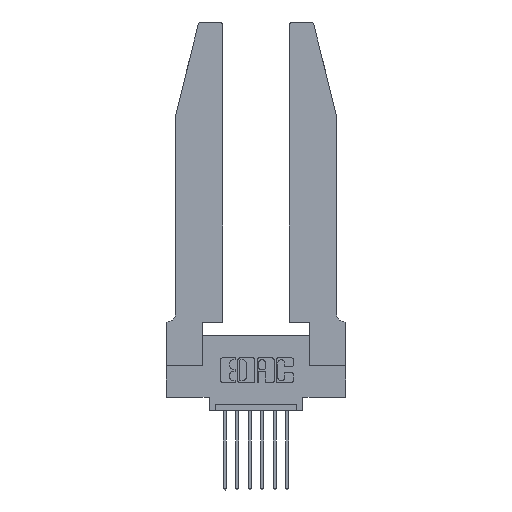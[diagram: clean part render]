
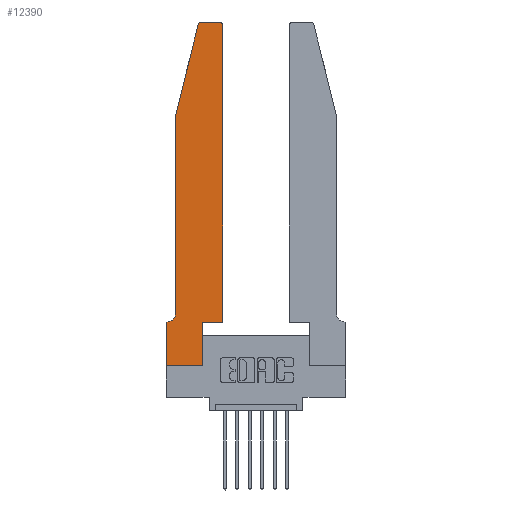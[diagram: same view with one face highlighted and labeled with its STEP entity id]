
A CAD part, top view. The second image highlights one B-rep face of the part: STEP entity #12390.
In plain terms, the highlighted planar face has unit normal (0, 0, 1).
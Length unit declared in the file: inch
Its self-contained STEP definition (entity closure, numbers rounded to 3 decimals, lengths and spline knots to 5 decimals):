
#160 = CARTESIAN_POINT ( 'NONE',  ( 0., 0.35, 0.37 ) ) ;
#162 = DIRECTION ( 'NONE',  ( -1., 0., 0. ) ) ;
#204 = PLANE ( 'NONE',  #5312 ) ;
#361 = DIRECTION ( 'NONE',  ( 1., 0., 0. ) ) ;
#409 = DIRECTION ( 'NONE',  ( 0., 0., 1. ) ) ;
#435 = VERTEX_POINT ( 'NONE', #12884 ) ;
#530 = CIRCLE ( 'NONE', #12871, 0.03 ) ;
#577 = DIRECTION ( 'NONE',  ( 1., 0., 0. ) ) ;
#799 = VERTEX_POINT ( 'NONE', #11457 ) ;
#1276 = LINE ( 'NONE', #7693, #9684 ) ;
#1311 = DIRECTION ( 'NONE',  ( -1., 0., 0. ) ) ;
#1637 = CARTESIAN_POINT ( 'NONE',  ( 0.284, 2.72, 0.37 ) ) ;
#1907 = ORIENTED_EDGE ( 'NONE', *, *, #7547, .T. ) ;
#2200 = VERTEX_POINT ( 'NONE', #2783 ) ;
#2266 = ORIENTED_EDGE ( 'NONE', *, *, #13866, .T. ) ;
#2279 = CIRCLE ( 'NONE', #2395, 0.07 ) ;
#2322 = VECTOR ( 'NONE', #10200, 39.37008 ) ;
#2341 = LINE ( 'NONE', #8963, #13403 ) ;
#2395 = AXIS2_PLACEMENT_3D ( 'NONE', #3370, #12209, #4284 ) ;
#2571 = EDGE_CURVE ( 'NONE', #3270, #6875, #530, .T. ) ;
#2683 = LINE ( 'NONE', #4864, #9753 ) ;
#2771 = DIRECTION ( 'NONE',  ( 1., 0., 0. ) ) ;
#2783 = CARTESIAN_POINT ( 'NONE',  ( 0.0055, 0.35, 0.37 ) ) ;
#3173 = VERTEX_POINT ( 'NONE', #13539 ) ;
#3248 = CARTESIAN_POINT ( 'NONE',  ( 0.4205, 2.75, 0.37 ) ) ;
#3270 = VERTEX_POINT ( 'NONE', #7578 ) ;
#3309 = CARTESIAN_POINT ( 'NONE',  ( 0., 0., 0.37 ) ) ;
#3370 = CARTESIAN_POINT ( 'NONE',  ( 0.0055, 0.42, 0.37 ) ) ;
#3454 = CARTESIAN_POINT ( 'NONE',  ( 0.0755, 0.42, 0.37 ) ) ;
#3624 = VECTOR ( 'NONE', #6893, 39.37008 ) ;
#3678 = CARTESIAN_POINT ( 'NONE',  ( 0., 0., 0.37 ) ) ;
#4079 = CARTESIAN_POINT ( 'NONE',  ( 0.0755, 2., 0.37 ) ) ;
#4284 = DIRECTION ( 'NONE',  ( -1., 0., 0. ) ) ;
#4397 = VECTOR ( 'NONE', #1311, 39.37008 ) ;
#4595 = DIRECTION ( 'NONE',  ( 1., 0., 0. ) ) ;
#4669 = EDGE_CURVE ( 'NONE', #2200, #3173, #7354, .T. ) ;
#4854 = VERTEX_POINT ( 'NONE', #3678 ) ;
#4864 = CARTESIAN_POINT ( 'NONE',  ( 0.4505, 0.35, 0.37 ) ) ;
#4888 = CARTESIAN_POINT ( 'NONE',  ( 0.4205, 2.72, 0.37 ) ) ;
#4927 = EDGE_CURVE ( 'NONE', #435, #7737, #2683, .T. ) ;
#5223 = VECTOR ( 'NONE', #4595, 39.37008 ) ;
#5266 = ORIENTED_EDGE ( 'NONE', *, *, #9468, .T. ) ;
#5312 = AXIS2_PLACEMENT_3D ( 'NONE', #160, #10130, #11325 ) ;
#5315 = LINE ( 'NONE', #10789, #8556 ) ;
#5510 = EDGE_CURVE ( 'NONE', #3173, #4854, #10440, .T. ) ;
#5637 = ORIENTED_EDGE ( 'NONE', *, *, #2571, .T. ) ;
#5814 = ORIENTED_EDGE ( 'NONE', *, *, #4927, .T. ) ;
#6471 = VERTEX_POINT ( 'NONE', #3248 ) ;
#6473 = ORIENTED_EDGE ( 'NONE', *, *, #7087, .T. ) ;
#6847 = CARTESIAN_POINT ( 'NONE',  ( 0.4505, 0.35, 0.37 ) ) ;
#6875 = VERTEX_POINT ( 'NONE', #13469 ) ;
#6893 = DIRECTION ( 'NONE',  ( 0., 1., 0. ) ) ;
#7062 = FACE_OUTER_BOUND ( 'NONE', #13129, .T. ) ;
#7087 = EDGE_CURVE ( 'NONE', #9486, #2200, #2279, .T. ) ;
#7101 = CIRCLE ( 'NONE', #13551, 0.03 ) ;
#7314 = ORIENTED_EDGE ( 'NONE', *, *, #9556, .T. ) ;
#7354 = LINE ( 'NONE', #7534, #4397 ) ;
#7426 = LINE ( 'NONE', #6847, #3624 ) ;
#7534 = CARTESIAN_POINT ( 'NONE',  ( 0.0755, 0.35, 0.37 ) ) ;
#7547 = EDGE_CURVE ( 'NONE', #7737, #10985, #7426, .T. ) ;
#7578 = CARTESIAN_POINT ( 'NONE',  ( 0.284, 2.75, 0.37 ) ) ;
#7693 = CARTESIAN_POINT ( 'NONE',  ( 0.2605, 2.75, 0.37 ) ) ;
#7723 = EDGE_CURVE ( 'NONE', #8467, #9486, #11390, .T. ) ;
#7737 = VERTEX_POINT ( 'NONE', #10017 ) ;
#7788 = LINE ( 'NONE', #3309, #5223 ) ;
#7909 = DIRECTION ( 'NONE',  ( -0.239, -0.971, 0. ) ) ;
#8229 = DIRECTION ( 'NONE',  ( 0., 0., 1. ) ) ;
#8467 = VERTEX_POINT ( 'NONE', #10449 ) ;
#8556 = VECTOR ( 'NONE', #13033, 39.37008 ) ;
#8605 = ORIENTED_EDGE ( 'NONE', *, *, #4669, .T. ) ;
#8676 = ORIENTED_EDGE ( 'NONE', *, *, #12314, .T. ) ;
#8781 = ORIENTED_EDGE ( 'NONE', *, *, #5510, .T. ) ;
#8963 = CARTESIAN_POINT ( 'NONE',  ( 0.0755, 2., 0.37 ) ) ;
#9336 = ORIENTED_EDGE ( 'NONE', *, *, #10871, .T. ) ;
#9468 = EDGE_CURVE ( 'NONE', #6471, #3270, #1276, .T. ) ;
#9486 = VERTEX_POINT ( 'NONE', #3454 ) ;
#9556 = EDGE_CURVE ( 'NONE', #4854, #799, #7788, .T. ) ;
#9684 = VECTOR ( 'NONE', #162, 39.37008 ) ;
#9753 = VECTOR ( 'NONE', #577, 39.37008 ) ;
#10017 = CARTESIAN_POINT ( 'NONE',  ( 0.4505, 0.35, 0.37 ) ) ;
#10130 = DIRECTION ( 'NONE',  ( 0., 0., 1. ) ) ;
#10200 = DIRECTION ( 'NONE',  ( 0., -1., 0. ) ) ;
#10440 = LINE ( 'NONE', #13397, #2322 ) ;
#10449 = CARTESIAN_POINT ( 'NONE',  ( 0.0755, 2., 0.37 ) ) ;
#10789 = CARTESIAN_POINT ( 'NONE',  ( 0.2865, 0.35, 0.37 ) ) ;
#10871 = EDGE_CURVE ( 'NONE', #10985, #6471, #7101, .T. ) ;
#10985 = VERTEX_POINT ( 'NONE', #13747 ) ;
#11325 = DIRECTION ( 'NONE',  ( 1., 0., 0. ) ) ;
#11390 = LINE ( 'NONE', #4079, #14145 ) ;
#11457 = CARTESIAN_POINT ( 'NONE',  ( 0.2865, 0., 0.37 ) ) ;
#11794 = DIRECTION ( 'NONE',  ( 0., -1., 0. ) ) ;
#12209 = DIRECTION ( 'NONE',  ( 0., 0., -1. ) ) ;
#12314 = EDGE_CURVE ( 'NONE', #799, #435, #5315, .T. ) ;
#12390 = ADVANCED_FACE ( 'NONE', ( #7062 ), #204, .T. ) ;
#12871 = AXIS2_PLACEMENT_3D ( 'NONE', #1637, #8229, #2771 ) ;
#12884 = CARTESIAN_POINT ( 'NONE',  ( 0.2865, 0.35, 0.37 ) ) ;
#13033 = DIRECTION ( 'NONE',  ( 0., 1., 0. ) ) ;
#13129 = EDGE_LOOP ( 'NONE', ( #5266, #5637, #2266, #14111, #6473, #8605, #8781, #7314, #8676, #5814, #1907, #9336 ) ) ;
#13397 = CARTESIAN_POINT ( 'NONE',  ( 0., 0., 0.37 ) ) ;
#13403 = VECTOR ( 'NONE', #7909, 39.37008 ) ;
#13469 = CARTESIAN_POINT ( 'NONE',  ( 0.25487, 2.72718, 0.37 ) ) ;
#13539 = CARTESIAN_POINT ( 'NONE',  ( 0., 0.35, 0.37 ) ) ;
#13551 = AXIS2_PLACEMENT_3D ( 'NONE', #4888, #409, #361 ) ;
#13747 = CARTESIAN_POINT ( 'NONE',  ( 0.4505, 2.72, 0.37 ) ) ;
#13866 = EDGE_CURVE ( 'NONE', #6875, #8467, #2341, .T. ) ;
#14111 = ORIENTED_EDGE ( 'NONE', *, *, #7723, .T. ) ;
#14145 = VECTOR ( 'NONE', #11794, 39.37008 ) ;
